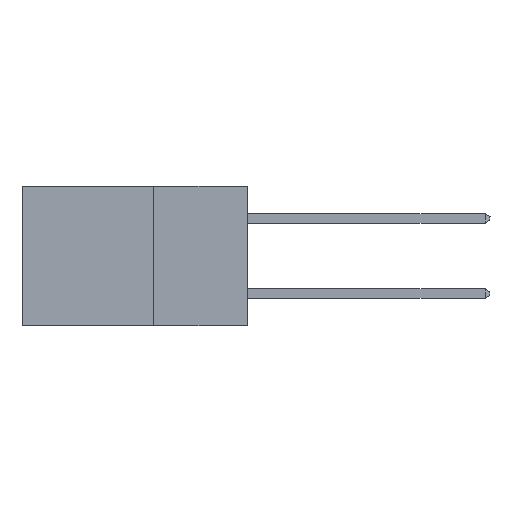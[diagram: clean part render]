
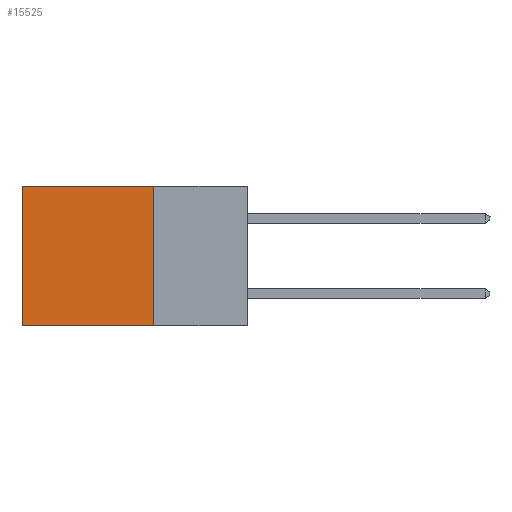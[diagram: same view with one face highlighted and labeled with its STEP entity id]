
A CAD part, left-side view. The second image highlights one B-rep face of the part: STEP entity #15525.
In plain terms, the highlighted planar face has unit normal (-1, 0, 0).
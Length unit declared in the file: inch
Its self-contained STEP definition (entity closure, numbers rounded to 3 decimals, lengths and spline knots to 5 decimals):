
#49 = CARTESIAN_POINT ( 'NONE',  ( 0.298, 0.25, 0. ) ) ;
#1038 = VECTOR ( 'NONE', #12189, 39.37008 ) ;
#1553 = CARTESIAN_POINT ( 'NONE',  ( 0.298, 0.25, 0. ) ) ;
#2495 = VECTOR ( 'NONE', #14119, 39.37008 ) ;
#4302 = VERTEX_POINT ( 'NONE', #28261 ) ;
#4589 = PLANE ( 'NONE',  #30426 ) ;
#5911 = LINE ( 'NONE', #1553, #17605 ) ;
#6005 = EDGE_LOOP ( 'NONE', ( #19517, #6572, #30184, #19473 ) ) ;
#6572 = ORIENTED_EDGE ( 'NONE', *, *, #10401, .F. ) ;
#7009 = DIRECTION ( 'NONE',  ( 0., 0., -1. ) ) ;
#7279 = VERTEX_POINT ( 'NONE', #20498 ) ;
#7543 = VERTEX_POINT ( 'NONE', #12485 ) ;
#8055 = FACE_OUTER_BOUND ( 'NONE', #6005, .T. ) ;
#8674 = DIRECTION ( 'NONE',  ( 0., 1., 0. ) ) ;
#8825 = EDGE_CURVE ( 'NONE', #7279, #4302, #10159, .T. ) ;
#10159 = LINE ( 'NONE', #28888, #1038 ) ;
#10401 = EDGE_CURVE ( 'NONE', #4302, #7543, #16825, .T. ) ;
#12189 = DIRECTION ( 'NONE',  ( 0., 0., -1. ) ) ;
#12485 = CARTESIAN_POINT ( 'NONE',  ( 0.298, 0.6, -0.37 ) ) ;
#13861 = EDGE_CURVE ( 'NONE', #7279, #22484, #5911, .T. ) ;
#14119 = DIRECTION ( 'NONE',  ( 0., 1., 0. ) ) ;
#15525 = ADVANCED_FACE ( 'NONE', ( #8055 ), #4589, .F. ) ;
#16437 = DIRECTION ( 'NONE',  ( 0., 0., -1. ) ) ;
#16825 = LINE ( 'NONE', #28614, #2495 ) ;
#17082 = EDGE_CURVE ( 'NONE', #22484, #7543, #24578, .T. ) ;
#17605 = VECTOR ( 'NONE', #8674, 39.37008 ) ;
#18192 = VECTOR ( 'NONE', #16437, 39.37008 ) ;
#19342 = DIRECTION ( 'NONE',  ( 1., 0., 0. ) ) ;
#19473 = ORIENTED_EDGE ( 'NONE', *, *, #13861, .T. ) ;
#19517 = ORIENTED_EDGE ( 'NONE', *, *, #17082, .T. ) ;
#20498 = CARTESIAN_POINT ( 'NONE',  ( 0.298, 0.25, 0. ) ) ;
#22484 = VERTEX_POINT ( 'NONE', #26715 ) ;
#24578 = LINE ( 'NONE', #30820, #18192 ) ;
#26715 = CARTESIAN_POINT ( 'NONE',  ( 0.298, 0.6, 0. ) ) ;
#28261 = CARTESIAN_POINT ( 'NONE',  ( 0.298, 0.25, -0.37 ) ) ;
#28614 = CARTESIAN_POINT ( 'NONE',  ( 0.298, 0.25, -0.37 ) ) ;
#28888 = CARTESIAN_POINT ( 'NONE',  ( 0.298, 0.25, 0. ) ) ;
#30184 = ORIENTED_EDGE ( 'NONE', *, *, #8825, .F. ) ;
#30426 = AXIS2_PLACEMENT_3D ( 'NONE', #49, #19342, #7009 ) ;
#30820 = CARTESIAN_POINT ( 'NONE',  ( 0.298, 0.6, 0. ) ) ;
